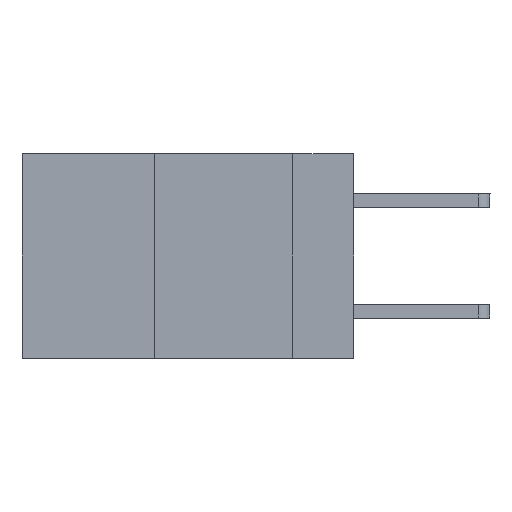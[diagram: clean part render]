
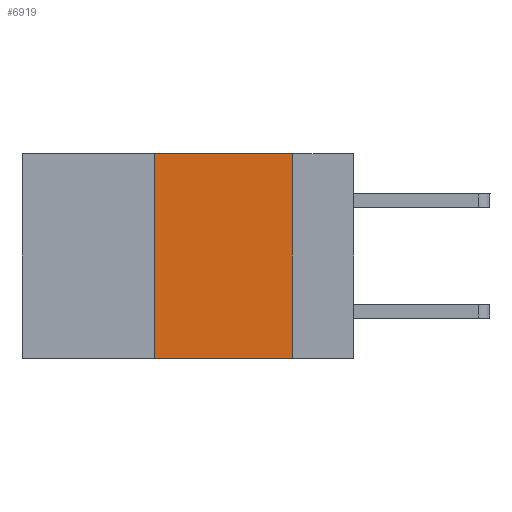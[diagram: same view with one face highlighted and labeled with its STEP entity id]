
A CAD part, left-side view. The second image highlights one B-rep face of the part: STEP entity #6919.
In plain terms, the highlighted planar face has unit normal (-1, 0, 0).
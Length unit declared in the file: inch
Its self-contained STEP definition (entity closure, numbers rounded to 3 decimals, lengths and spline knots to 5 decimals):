
#224 = DIRECTION ( 'NONE',  ( 0., -1., 0. ) ) ;
#755 = LINE ( 'NONE', #12958, #2312 ) ;
#953 = VECTOR ( 'NONE', #4794, 39.37008 ) ;
#1002 = EDGE_CURVE ( 'NONE', #11403, #5454, #8695, .T. ) ;
#1840 = ORIENTED_EDGE ( 'NONE', *, *, #1002, .F. ) ;
#2312 = VECTOR ( 'NONE', #10729, 39.37008 ) ;
#2455 = DIRECTION ( 'NONE',  ( 1., 0., 0. ) ) ;
#2522 = DIRECTION ( 'NONE',  ( 0., 0., -1. ) ) ;
#2597 = LINE ( 'NONE', #6038, #7069 ) ;
#3222 = VERTEX_POINT ( 'NONE', #14362 ) ;
#3553 = CARTESIAN_POINT ( 'NONE',  ( 0., 0.6, 0. ) ) ;
#4162 = ORIENTED_EDGE ( 'NONE', *, *, #8722, .F. ) ;
#4429 = ORIENTED_EDGE ( 'NONE', *, *, #13308, .F. ) ;
#4794 = DIRECTION ( 'NONE',  ( 0., -1., 0. ) ) ;
#4852 = VERTEX_POINT ( 'NONE', #6287 ) ;
#5454 = VERTEX_POINT ( 'NONE', #12061 ) ;
#5546 = AXIS2_PLACEMENT_3D ( 'NONE', #3553, #2455, #2522 ) ;
#6008 = ORIENTED_EDGE ( 'NONE', *, *, #13348, .T. ) ;
#6038 = CARTESIAN_POINT ( 'NONE',  ( 0., 0.6, 0. ) ) ;
#6174 = VECTOR ( 'NONE', #9665, 39.37008 ) ;
#6217 = CARTESIAN_POINT ( 'NONE',  ( 0., 0.11, 0. ) ) ;
#6287 = CARTESIAN_POINT ( 'NONE',  ( 0., 0.36, 0. ) ) ;
#6919 = ADVANCED_FACE ( 'NONE', ( #11613 ), #13671, .F. ) ;
#7069 = VECTOR ( 'NONE', #224, 39.37008 ) ;
#8695 = LINE ( 'NONE', #11077, #6174 ) ;
#8722 = EDGE_CURVE ( 'NONE', #3222, #4852, #755, .T. ) ;
#9229 = CARTESIAN_POINT ( 'NONE',  ( 0., 0.6, -0.37 ) ) ;
#9665 = DIRECTION ( 'NONE',  ( 0., 0., -1. ) ) ;
#10729 = DIRECTION ( 'NONE',  ( 0., 0., 1. ) ) ;
#11077 = CARTESIAN_POINT ( 'NONE',  ( 0., 0.11, 0. ) ) ;
#11403 = VERTEX_POINT ( 'NONE', #6217 ) ;
#11613 = FACE_OUTER_BOUND ( 'NONE', #12367, .T. ) ;
#12061 = CARTESIAN_POINT ( 'NONE',  ( 0., 0.11, -0.37 ) ) ;
#12367 = EDGE_LOOP ( 'NONE', ( #1840, #4429, #4162, #6008 ) ) ;
#12958 = CARTESIAN_POINT ( 'NONE',  ( 0., 0.36, 0. ) ) ;
#13308 = EDGE_CURVE ( 'NONE', #4852, #11403, #2597, .T. ) ;
#13348 = EDGE_CURVE ( 'NONE', #3222, #5454, #13744, .T. ) ;
#13671 = PLANE ( 'NONE',  #5546 ) ;
#13744 = LINE ( 'NONE', #9229, #953 ) ;
#14362 = CARTESIAN_POINT ( 'NONE',  ( 0., 0.36, -0.37 ) ) ;
